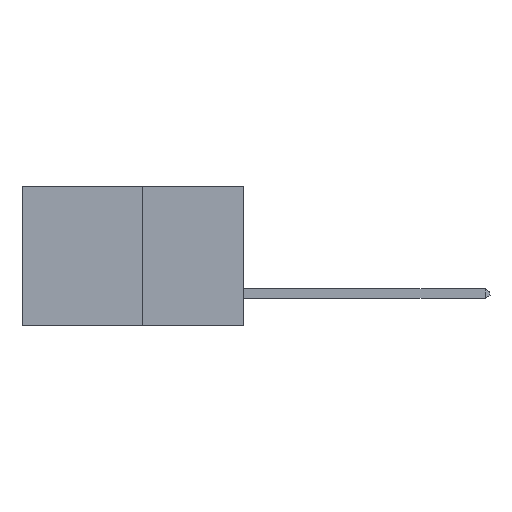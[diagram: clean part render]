
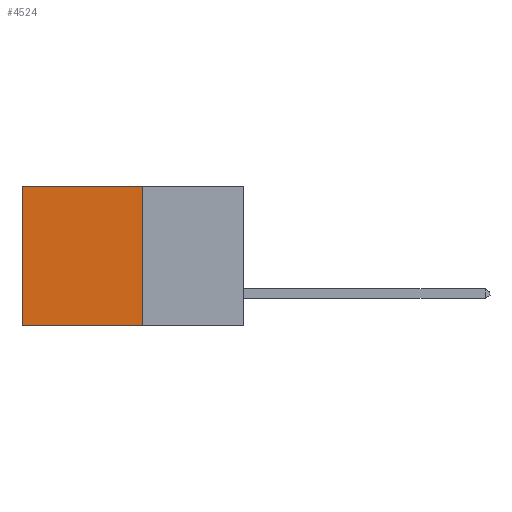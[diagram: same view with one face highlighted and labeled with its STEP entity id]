
A CAD part, left-side view. The second image highlights one B-rep face of the part: STEP entity #4524.
In plain terms, the highlighted planar face has unit normal (-1, 0, 0).
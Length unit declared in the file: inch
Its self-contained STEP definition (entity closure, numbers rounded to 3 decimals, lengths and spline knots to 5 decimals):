
#145 = CARTESIAN_POINT ( 'NONE',  ( 0.277, 0.27, 0. ) ) ;
#857 = CARTESIAN_POINT ( 'NONE',  ( 0.277, 0.59, -0.37 ) ) ;
#1149 = EDGE_LOOP ( 'NONE', ( #8324, #3804, #7537, #5002 ) ) ;
#1537 = LINE ( 'NONE', #3713, #4154 ) ;
#2284 = DIRECTION ( 'NONE',  ( 0., 0., -1. ) ) ;
#2721 = LINE ( 'NONE', #7502, #11085 ) ;
#3032 = DIRECTION ( 'NONE',  ( 1., 0., 0. ) ) ;
#3153 = VERTEX_POINT ( 'NONE', #13399 ) ;
#3395 = CARTESIAN_POINT ( 'NONE',  ( 0.277, 0.27, -0.37 ) ) ;
#3713 = CARTESIAN_POINT ( 'NONE',  ( 0.277, 0.27, -0.37 ) ) ;
#3766 = DIRECTION ( 'NONE',  ( 0., 1., 0. ) ) ;
#3804 = ORIENTED_EDGE ( 'NONE', *, *, #7891, .F. ) ;
#3925 = CARTESIAN_POINT ( 'NONE',  ( 0.277, 0.59, -0.37 ) ) ;
#4066 = FACE_OUTER_BOUND ( 'NONE', #1149, .T. ) ;
#4154 = VECTOR ( 'NONE', #3766, 39.37008 ) ;
#4524 = ADVANCED_FACE ( 'NONE', ( #4066 ), #8403, .F. ) ;
#4687 = EDGE_CURVE ( 'NONE', #9513, #3153, #2721, .T. ) ;
#5002 = ORIENTED_EDGE ( 'NONE', *, *, #7580, .T. ) ;
#5671 = VERTEX_POINT ( 'NONE', #11632 ) ;
#5707 = VECTOR ( 'NONE', #6297, 39.37008 ) ;
#6280 = AXIS2_PLACEMENT_3D ( 'NONE', #3395, #3032, #7905 ) ;
#6297 = DIRECTION ( 'NONE',  ( 0., 1., 0. ) ) ;
#7502 = CARTESIAN_POINT ( 'NONE',  ( 0.277, 0.27, -0.37 ) ) ;
#7537 = ORIENTED_EDGE ( 'NONE', *, *, #4687, .F. ) ;
#7580 = EDGE_CURVE ( 'NONE', #9513, #5671, #8515, .T. ) ;
#7891 = EDGE_CURVE ( 'NONE', #3153, #8193, #1537, .T. ) ;
#7905 = DIRECTION ( 'NONE',  ( 0., 0., -1. ) ) ;
#8193 = VERTEX_POINT ( 'NONE', #857 ) ;
#8324 = ORIENTED_EDGE ( 'NONE', *, *, #12689, .T. ) ;
#8403 = PLANE ( 'NONE',  #6280 ) ;
#8515 = LINE ( 'NONE', #145, #5707 ) ;
#8704 = CARTESIAN_POINT ( 'NONE',  ( 0.277, 0.27, 0. ) ) ;
#9513 = VERTEX_POINT ( 'NONE', #8704 ) ;
#10693 = LINE ( 'NONE', #3925, #13171 ) ;
#11085 = VECTOR ( 'NONE', #2284, 39.37008 ) ;
#11220 = DIRECTION ( 'NONE',  ( 0., 0., -1. ) ) ;
#11632 = CARTESIAN_POINT ( 'NONE',  ( 0.277, 0.59, 0. ) ) ;
#12689 = EDGE_CURVE ( 'NONE', #5671, #8193, #10693, .T. ) ;
#13171 = VECTOR ( 'NONE', #11220, 39.37008 ) ;
#13399 = CARTESIAN_POINT ( 'NONE',  ( 0.277, 0.27, -0.37 ) ) ;
